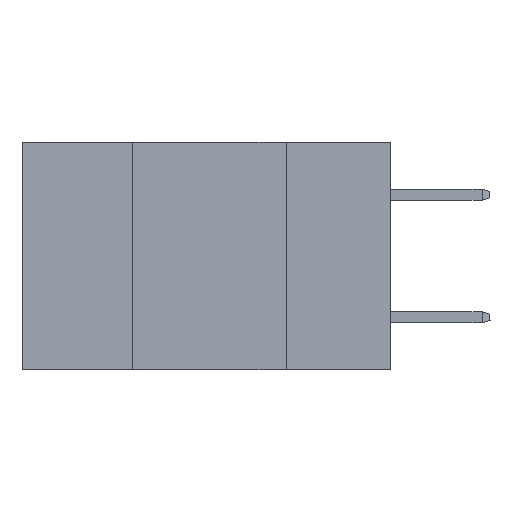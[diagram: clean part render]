
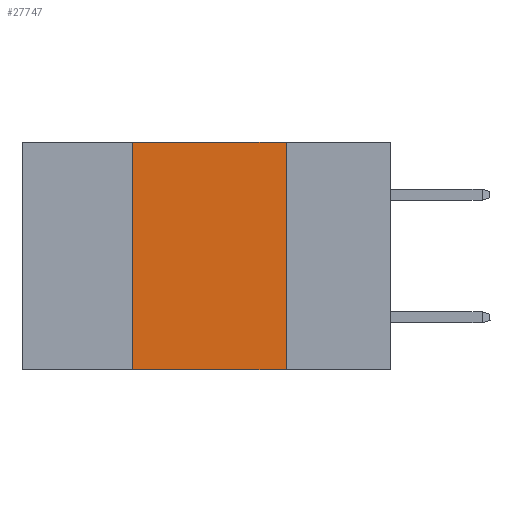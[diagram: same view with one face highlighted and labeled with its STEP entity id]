
A CAD part, left-side view. The second image highlights one B-rep face of the part: STEP entity #27747.
In plain terms, the highlighted planar face has unit normal (-1, 0, 0).
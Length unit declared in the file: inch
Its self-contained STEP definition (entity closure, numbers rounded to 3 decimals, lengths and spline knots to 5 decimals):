
#147 = EDGE_CURVE ( 'NONE', #14463, #11519, #30885, .T. ) ;
#374 = ORIENTED_EDGE ( 'NONE', *, *, #22919, .F. ) ;
#511 = LINE ( 'NONE', #12431, #31183 ) ;
#1675 = ORIENTED_EDGE ( 'NONE', *, *, #23947, .F. ) ;
#1903 = CARTESIAN_POINT ( 'NONE',  ( 0., 0.42, -0.37 ) ) ;
#2156 = VECTOR ( 'NONE', #23561, 39.37008 ) ;
#5536 = LINE ( 'NONE', #5698, #24174 ) ;
#5698 = CARTESIAN_POINT ( 'NONE',  ( 0., 0.17, 0. ) ) ;
#6049 = LINE ( 'NONE', #28779, #2156 ) ;
#6055 = PLANE ( 'NONE',  #31039 ) ;
#6214 = CARTESIAN_POINT ( 'NONE',  ( 0., 0.6, 0. ) ) ;
#8117 = EDGE_LOOP ( 'NONE', ( #1675, #374, #18982, #22352 ) ) ;
#8164 = EDGE_CURVE ( 'NONE', #14463, #24630, #511, .T. ) ;
#9557 = CARTESIAN_POINT ( 'NONE',  ( 0., 0.17, -0.37 ) ) ;
#11270 = FACE_OUTER_BOUND ( 'NONE', #8117, .T. ) ;
#11403 = VECTOR ( 'NONE', #26161, 39.37008 ) ;
#11519 = VERTEX_POINT ( 'NONE', #24675 ) ;
#12431 = CARTESIAN_POINT ( 'NONE',  ( 0., 0.6, -0.37 ) ) ;
#14463 = VERTEX_POINT ( 'NONE', #1903 ) ;
#15391 = VERTEX_POINT ( 'NONE', #29635 ) ;
#18458 = CARTESIAN_POINT ( 'NONE',  ( 0., 0.42, 0. ) ) ;
#18982 = ORIENTED_EDGE ( 'NONE', *, *, #147, .F. ) ;
#20121 = DIRECTION ( 'NONE',  ( 0., -1., 0. ) ) ;
#22352 = ORIENTED_EDGE ( 'NONE', *, *, #8164, .T. ) ;
#22801 = DIRECTION ( 'NONE',  ( 1., 0., 0. ) ) ;
#22919 = EDGE_CURVE ( 'NONE', #11519, #15391, #6049, .T. ) ;
#23529 = DIRECTION ( 'NONE',  ( 0., 0., -1. ) ) ;
#23561 = DIRECTION ( 'NONE',  ( 0., -1., 0. ) ) ;
#23729 = DIRECTION ( 'NONE',  ( 0., 0., -1. ) ) ;
#23947 = EDGE_CURVE ( 'NONE', #15391, #24630, #5536, .T. ) ;
#24174 = VECTOR ( 'NONE', #23529, 39.37008 ) ;
#24630 = VERTEX_POINT ( 'NONE', #9557 ) ;
#24675 = CARTESIAN_POINT ( 'NONE',  ( 0., 0.42, 0. ) ) ;
#26161 = DIRECTION ( 'NONE',  ( 0., 0., 1. ) ) ;
#27747 = ADVANCED_FACE ( 'NONE', ( #11270 ), #6055, .F. ) ;
#28779 = CARTESIAN_POINT ( 'NONE',  ( 0., 0.6, 0. ) ) ;
#29635 = CARTESIAN_POINT ( 'NONE',  ( 0., 0.17, 0. ) ) ;
#30885 = LINE ( 'NONE', #18458, #11403 ) ;
#31039 = AXIS2_PLACEMENT_3D ( 'NONE', #6214, #22801, #23729 ) ;
#31183 = VECTOR ( 'NONE', #20121, 39.37008 ) ;
